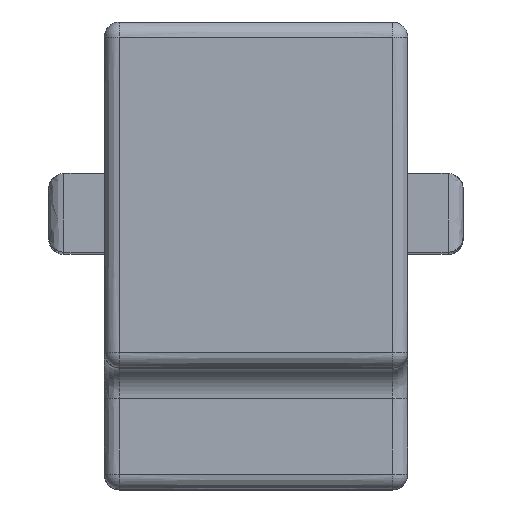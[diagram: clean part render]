
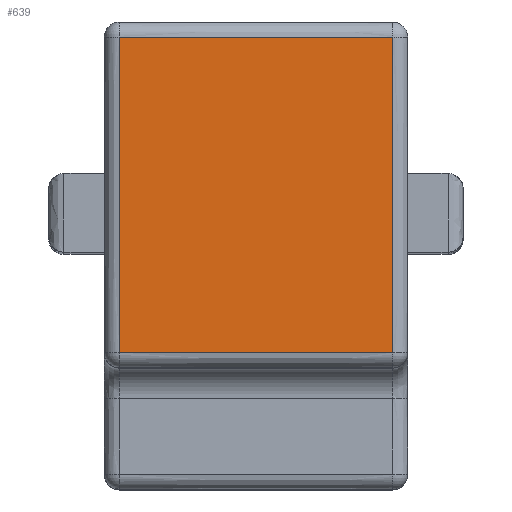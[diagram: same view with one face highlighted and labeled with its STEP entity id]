
A CAD part, top view. The second image highlights one B-rep face of the part: STEP entity #639.
In plain terms, the highlighted planar face has unit normal (0, 0, 1).
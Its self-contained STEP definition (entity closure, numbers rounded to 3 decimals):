
#8 = CARTESIAN_POINT ( 'NONE',  ( 4.75, -0.26, -1.526 ) ) ;
#99 = EDGE_CURVE ( 'NONE', #3066, #1463, #2748, .T. ) ;
#134 = CARTESIAN_POINT ( 'NONE',  ( -4.275, -10.615, -1.526 ) ) ;
#229 = EDGE_CURVE ( 'NONE', #1864, #2864, #2193, .T. ) ;
#274 = DIRECTION ( 'NONE',  ( 0., 0., -1. ) ) ;
#323 = CARTESIAN_POINT ( 'NONE',  ( 4.275, -10.615, -1.526 ) ) ;
#332 = CARTESIAN_POINT ( 'NONE',  ( 1.425, -0.735, -1.526 ) ) ;
#368 = EDGE_CURVE ( 'NONE', #2864, #3066, #2579, .T. ) ;
#590 = ORIENTED_EDGE ( 'NONE', *, *, #2101, .T. ) ;
#639 = ADVANCED_FACE ( 'NONE', ( #1519 ), #1998, .F. ) ;
#642 = ORIENTED_EDGE ( 'NONE', *, *, #368, .T. ) ;
#726 = CARTESIAN_POINT ( 'NONE',  ( 4.275, -7.321, -1.526 ) ) ;
#808 = B_SPLINE_CURVE_WITH_KNOTS ( 'NONE', 3,
 ( #134, #1361, #1863, #2347 ),
 .UNSPECIFIED., .F., .F.,
 ( 4, 4 ),
 ( 0., 1. ),
 .UNSPECIFIED. ) ;
#1127 = CARTESIAN_POINT ( 'NONE',  ( 4.275, -0.735, -1.526 ) ) ;
#1163 = CARTESIAN_POINT ( 'NONE',  ( -4.275, -0.735, -1.526 ) ) ;
#1223 = CARTESIAN_POINT ( 'NONE',  ( -4.275, -10.615, -1.526 ) ) ;
#1281 = AXIS2_PLACEMENT_3D ( 'NONE', #8, #274, #2018 ) ;
#1361 = CARTESIAN_POINT ( 'NONE',  ( -1.425, -10.615, -1.526 ) ) ;
#1463 = VERTEX_POINT ( 'NONE', #2304 ) ;
#1519 = FACE_OUTER_BOUND ( 'NONE', #2302, .T. ) ;
#1685 = CARTESIAN_POINT ( 'NONE',  ( 4.275, -10.615, -1.526 ) ) ;
#1863 = CARTESIAN_POINT ( 'NONE',  ( 1.425, -10.615, -1.526 ) ) ;
#1864 = VERTEX_POINT ( 'NONE', #323 ) ;
#1998 = PLANE ( 'NONE',  #1281 ) ;
#2018 = DIRECTION ( 'NONE',  ( 0., 1., 0. ) ) ;
#2101 = EDGE_CURVE ( 'NONE', #1463, #1864, #808, .T. ) ;
#2193 = B_SPLINE_CURVE_WITH_KNOTS ( 'NONE', 3,
 ( #1685, #726, #2979, #2461 ),
 .UNSPECIFIED., .F., .F.,
 ( 4, 4 ),
 ( 0., 1. ),
 .UNSPECIFIED. ) ;
#2205 = CARTESIAN_POINT ( 'NONE',  ( -4.275, -0.735, -1.526 ) ) ;
#2208 = ORIENTED_EDGE ( 'NONE', *, *, #229, .T. ) ;
#2235 = CARTESIAN_POINT ( 'NONE',  ( -4.275, -7.321, -1.526 ) ) ;
#2302 = EDGE_LOOP ( 'NONE', ( #642, #2348, #590, #2208 ) ) ;
#2304 = CARTESIAN_POINT ( 'NONE',  ( -4.275, -10.615, -1.526 ) ) ;
#2319 = CARTESIAN_POINT ( 'NONE',  ( -4.275, -0.735, -1.526 ) ) ;
#2347 = CARTESIAN_POINT ( 'NONE',  ( 4.275, -10.615, -1.526 ) ) ;
#2348 = ORIENTED_EDGE ( 'NONE', *, *, #99, .T. ) ;
#2461 = CARTESIAN_POINT ( 'NONE',  ( 4.275, -0.735, -1.526 ) ) ;
#2579 = B_SPLINE_CURVE_WITH_KNOTS ( 'NONE', 3,
 ( #1127, #332, #2870, #2319 ),
 .UNSPECIFIED., .F., .F.,
 ( 4, 4 ),
 ( 0., 1. ),
 .UNSPECIFIED. ) ;
#2748 = B_SPLINE_CURVE_WITH_KNOTS ( 'NONE', 3,
 ( #2205, #2968, #2235, #1223 ),
 .UNSPECIFIED., .F., .F.,
 ( 4, 4 ),
 ( 0., 1. ),
 .UNSPECIFIED. ) ;
#2864 = VERTEX_POINT ( 'NONE', #3118 ) ;
#2870 = CARTESIAN_POINT ( 'NONE',  ( -1.425, -0.735, -1.526 ) ) ;
#2968 = CARTESIAN_POINT ( 'NONE',  ( -4.275, -4.028, -1.526 ) ) ;
#2979 = CARTESIAN_POINT ( 'NONE',  ( 4.275, -4.028, -1.526 ) ) ;
#3066 = VERTEX_POINT ( 'NONE', #1163 ) ;
#3118 = CARTESIAN_POINT ( 'NONE',  ( 4.275, -0.735, -1.526 ) ) ;
